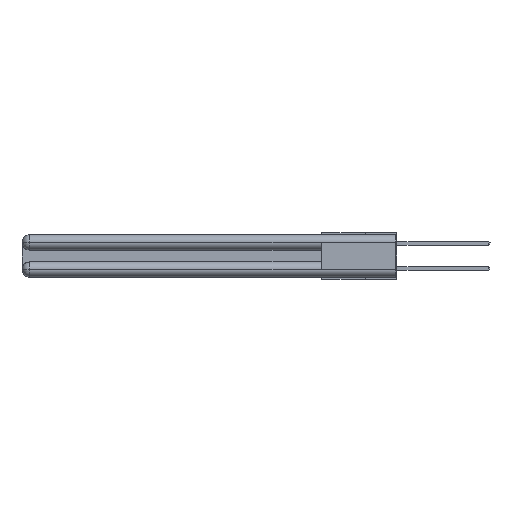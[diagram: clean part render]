
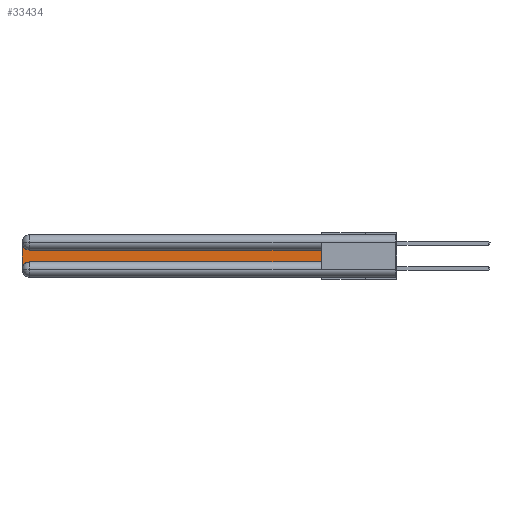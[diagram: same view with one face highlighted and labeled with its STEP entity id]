
A CAD part, left-side view. The second image highlights one B-rep face of the part: STEP entity #33434.
In plain terms, the highlighted planar face has unit normal (-1, 0, 0).
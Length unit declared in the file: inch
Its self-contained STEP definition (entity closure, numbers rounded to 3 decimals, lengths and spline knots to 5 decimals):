
#1989 = ORIENTED_EDGE ( 'NONE', *, *, #21921, .T. ) ;
#2393 = VERTEX_POINT ( 'NONE', #32264 ) ;
#2840 = VECTOR ( 'NONE', #6031, 39.37008 ) ;
#3066 = DIRECTION ( 'NONE',  ( 0., 0., -1. ) ) ;
#3132 = FACE_OUTER_BOUND ( 'NONE', #20072, .T. ) ;
#3872 = CIRCLE ( 'NONE', #18991, 0.06 ) ;
#3882 = EDGE_CURVE ( 'NONE', #2393, #27821, #27649, .T. ) ;
#4263 = VERTEX_POINT ( 'NONE', #22324 ) ;
#5131 = EDGE_CURVE ( 'NONE', #29965, #4263, #5818, .T. ) ;
#5818 = LINE ( 'NONE', #17210, #2840 ) ;
#6031 = DIRECTION ( 'NONE',  ( 0., 0., -1. ) ) ;
#6431 = CIRCLE ( 'NONE', #9156, 0.06 ) ;
#6631 = CARTESIAN_POINT ( 'NONE',  ( 0.075, 2.94, -0.0625 ) ) ;
#7698 = VECTOR ( 'NONE', #21724, 39.37008 ) ;
#8149 = VECTOR ( 'NONE', #27668, 39.37008 ) ;
#9156 = AXIS2_PLACEMENT_3D ( 'NONE', #30175, #19357, #3066 ) ;
#11924 = CARTESIAN_POINT ( 'NONE',  ( 0.075, 3., -0.1225 ) ) ;
#11929 = CARTESIAN_POINT ( 'NONE',  ( 0.075, 2.94, -0.1225 ) ) ;
#11954 = ORIENTED_EDGE ( 'NONE', *, *, #15429, .T. ) ;
#13685 = LINE ( 'NONE', #13793, #8149 ) ;
#13793 = CARTESIAN_POINT ( 'NONE',  ( 0.075, 0.6, -0.2175 ) ) ;
#14748 = ORIENTED_EDGE ( 'NONE', *, *, #3882, .T. ) ;
#14755 = LINE ( 'NONE', #18152, #21138 ) ;
#15429 = EDGE_CURVE ( 'NONE', #27821, #21639, #14755, .T. ) ;
#17210 = CARTESIAN_POINT ( 'NONE',  ( 0.075, 3., -0.2175 ) ) ;
#18152 = CARTESIAN_POINT ( 'NONE',  ( 0.075, 0.6, -0.1225 ) ) ;
#18561 = CARTESIAN_POINT ( 'NONE',  ( 0.075, 0.6, -0.1225 ) ) ;
#18991 = AXIS2_PLACEMENT_3D ( 'NONE', #6631, #23378, #31356 ) ;
#19357 = DIRECTION ( 'NONE',  ( 1., 0., 0. ) ) ;
#20072 = EDGE_LOOP ( 'NONE', ( #11954, #24017, #24909, #1989, #28984, #14748 ) ) ;
#21138 = VECTOR ( 'NONE', #28873, 39.37008 ) ;
#21472 = CARTESIAN_POINT ( 'NONE',  ( 0.075, 2.94, -0.2175 ) ) ;
#21639 = VERTEX_POINT ( 'NONE', #11929 ) ;
#21724 = DIRECTION ( 'NONE',  ( 0., 0., 1. ) ) ;
#21921 = EDGE_CURVE ( 'NONE', #4263, #31442, #6431, .T. ) ;
#22060 = CARTESIAN_POINT ( 'NONE',  ( 0.075, 0.6, -0.2175 ) ) ;
#22324 = CARTESIAN_POINT ( 'NONE',  ( 0.075, 3., -0.2775 ) ) ;
#23378 = DIRECTION ( 'NONE',  ( 1., 0., 0. ) ) ;
#24017 = ORIENTED_EDGE ( 'NONE', *, *, #24546, .T. ) ;
#24546 = EDGE_CURVE ( 'NONE', #21639, #29965, #3872, .T. ) ;
#24909 = ORIENTED_EDGE ( 'NONE', *, *, #5131, .T. ) ;
#25460 = EDGE_CURVE ( 'NONE', #31442, #2393, #13685, .T. ) ;
#27649 = LINE ( 'NONE', #22060, #7698 ) ;
#27668 = DIRECTION ( 'NONE',  ( 0., -1., 0. ) ) ;
#27821 = VERTEX_POINT ( 'NONE', #18561 ) ;
#28185 = PLANE ( 'NONE',  #32170 ) ;
#28873 = DIRECTION ( 'NONE',  ( 0., 1., 0. ) ) ;
#28984 = ORIENTED_EDGE ( 'NONE', *, *, #25460, .T. ) ;
#29965 = VERTEX_POINT ( 'NONE', #31198 ) ;
#30175 = CARTESIAN_POINT ( 'NONE',  ( 0.075, 2.94, -0.2775 ) ) ;
#30925 = DIRECTION ( 'NONE',  ( 1., 0., 0. ) ) ;
#31051 = DIRECTION ( 'NONE',  ( 0., 0., -1. ) ) ;
#31198 = CARTESIAN_POINT ( 'NONE',  ( 0.075, 3., -0.0625 ) ) ;
#31356 = DIRECTION ( 'NONE',  ( 0., 0., -1. ) ) ;
#31442 = VERTEX_POINT ( 'NONE', #21472 ) ;
#32170 = AXIS2_PLACEMENT_3D ( 'NONE', #11924, #30925, #31051 ) ;
#32264 = CARTESIAN_POINT ( 'NONE',  ( 0.075, 0.6, -0.2175 ) ) ;
#33434 = ADVANCED_FACE ( 'NONE', ( #3132 ), #28185, .F. ) ;
